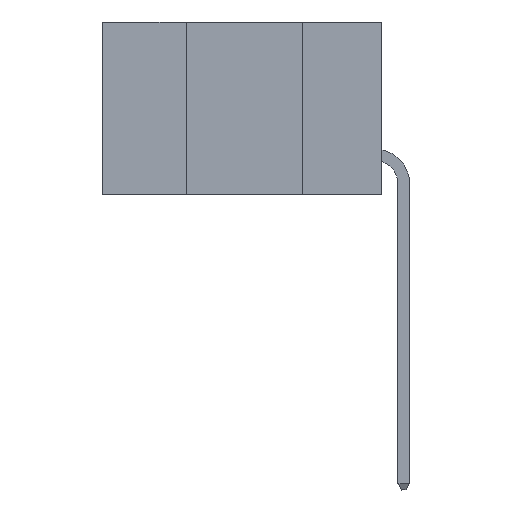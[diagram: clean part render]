
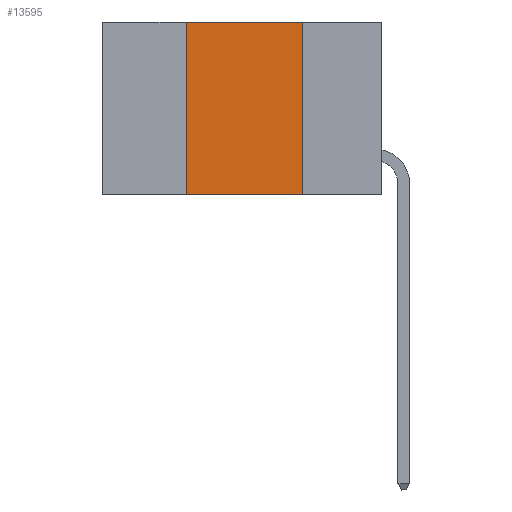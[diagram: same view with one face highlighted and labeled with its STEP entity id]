
A CAD part, left-side view. The second image highlights one B-rep face of the part: STEP entity #13595.
In plain terms, the highlighted planar face has unit normal (-1, 0, 0).
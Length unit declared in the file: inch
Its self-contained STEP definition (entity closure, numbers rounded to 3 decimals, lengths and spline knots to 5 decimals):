
#1611 = EDGE_CURVE ( 'NONE', #6041, #6344, #31324, .T. ) ;
#1764 = CARTESIAN_POINT ( 'NONE',  ( 0., 0.6, -0.37 ) ) ;
#2250 = CARTESIAN_POINT ( 'NONE',  ( 0., 0.17, 0. ) ) ;
#3089 = PLANE ( 'NONE',  #3339 ) ;
#3339 = AXIS2_PLACEMENT_3D ( 'NONE', #14909, #17393, #11463 ) ;
#4554 = CARTESIAN_POINT ( 'NONE',  ( 0., 0.17, -0.37 ) ) ;
#6041 = VERTEX_POINT ( 'NONE', #27657 ) ;
#6344 = VERTEX_POINT ( 'NONE', #4554 ) ;
#6807 = EDGE_CURVE ( 'NONE', #16919, #16452, #12721, .T. ) ;
#7629 = ORIENTED_EDGE ( 'NONE', *, *, #23203, .T. ) ;
#7688 = CARTESIAN_POINT ( 'NONE',  ( 0., 0.6, 0. ) ) ;
#7812 = VECTOR ( 'NONE', #23973, 39.37008 ) ;
#7984 = CARTESIAN_POINT ( 'NONE',  ( 0., 0.42, -0.37 ) ) ;
#8515 = LINE ( 'NONE', #7688, #14313 ) ;
#8693 = DIRECTION ( 'NONE',  ( 0., 0., 1. ) ) ;
#11463 = DIRECTION ( 'NONE',  ( 0., 0., -1. ) ) ;
#12721 = LINE ( 'NONE', #21291, #18926 ) ;
#13595 = ADVANCED_FACE ( 'NONE', ( #17249 ), #3089, .F. ) ;
#14313 = VECTOR ( 'NONE', #20370, 39.37008 ) ;
#14909 = CARTESIAN_POINT ( 'NONE',  ( 0., 0.6, 0. ) ) ;
#16452 = VERTEX_POINT ( 'NONE', #17430 ) ;
#16892 = ORIENTED_EDGE ( 'NONE', *, *, #18278, .F. ) ;
#16919 = VERTEX_POINT ( 'NONE', #7984 ) ;
#17249 = FACE_OUTER_BOUND ( 'NONE', #21714, .T. ) ;
#17393 = DIRECTION ( 'NONE',  ( 1., 0., 0. ) ) ;
#17430 = CARTESIAN_POINT ( 'NONE',  ( 0., 0.42, 0. ) ) ;
#18278 = EDGE_CURVE ( 'NONE', #16452, #6041, #8515, .T. ) ;
#18926 = VECTOR ( 'NONE', #8693, 39.37008 ) ;
#19520 = DIRECTION ( 'NONE',  ( 0., 0., -1. ) ) ;
#20142 = VECTOR ( 'NONE', #19520, 39.37008 ) ;
#20370 = DIRECTION ( 'NONE',  ( 0., -1., 0. ) ) ;
#21291 = CARTESIAN_POINT ( 'NONE',  ( 0., 0.42, 0. ) ) ;
#21714 = EDGE_LOOP ( 'NONE', ( #26722, #16892, #30312, #7629 ) ) ;
#23203 = EDGE_CURVE ( 'NONE', #16919, #6344, #24739, .T. ) ;
#23973 = DIRECTION ( 'NONE',  ( 0., -1., 0. ) ) ;
#24739 = LINE ( 'NONE', #1764, #7812 ) ;
#26722 = ORIENTED_EDGE ( 'NONE', *, *, #1611, .F. ) ;
#27657 = CARTESIAN_POINT ( 'NONE',  ( 0., 0.17, 0. ) ) ;
#30312 = ORIENTED_EDGE ( 'NONE', *, *, #6807, .F. ) ;
#31324 = LINE ( 'NONE', #2250, #20142 ) ;
